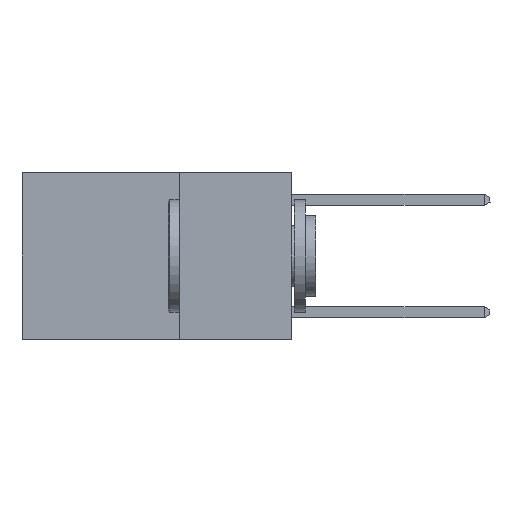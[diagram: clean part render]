
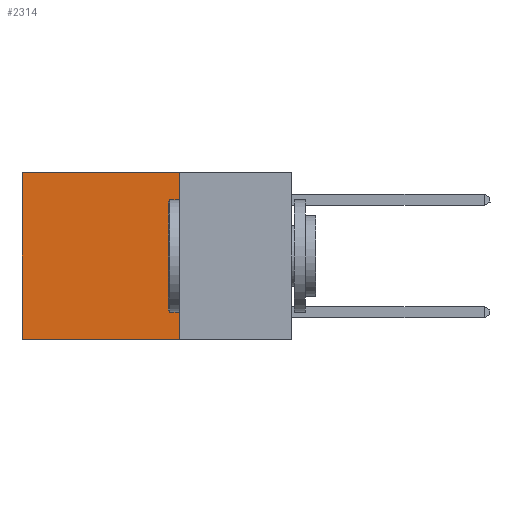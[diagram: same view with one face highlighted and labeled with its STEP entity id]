
A CAD part, left-side view. The second image highlights one B-rep face of the part: STEP entity #2314.
In plain terms, the highlighted planar face has unit normal (-1, 0, 0).
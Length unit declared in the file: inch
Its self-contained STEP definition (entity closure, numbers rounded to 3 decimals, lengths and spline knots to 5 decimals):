
#237 = PLANE ( 'NONE',  #12781 ) ;
#342 = CARTESIAN_POINT ( 'NONE',  ( 0.2625, 0.25, -0.37 ) ) ;
#918 = EDGE_CURVE ( 'NONE', #11127, #9048, #18905, .T. ) ;
#1229 = ORIENTED_EDGE ( 'NONE', *, *, #2737, .F. ) ;
#1987 = LINE ( 'NONE', #20059, #13210 ) ;
#2314 = ADVANCED_FACE ( 'NONE', ( #23925 ), #237, .F. ) ;
#2494 = ORIENTED_EDGE ( 'NONE', *, *, #918, .T. ) ;
#2737 = EDGE_CURVE ( 'NONE', #11127, #18868, #18816, .T. ) ;
#3712 = CARTESIAN_POINT ( 'NONE',  ( 0.2625, 0.25, -0.37 ) ) ;
#6930 = CARTESIAN_POINT ( 'NONE',  ( 0.2625, 0.25, 0. ) ) ;
#7854 = EDGE_CURVE ( 'NONE', #18868, #22643, #19022, .T. ) ;
#8993 = VECTOR ( 'NONE', #26523, 39.37008 ) ;
#9048 = VERTEX_POINT ( 'NONE', #21240 ) ;
#10449 = VECTOR ( 'NONE', #20209, 39.37008 ) ;
#10558 = VECTOR ( 'NONE', #26427, 39.37008 ) ;
#10932 = CARTESIAN_POINT ( 'NONE',  ( 0.2625, 0.6, -0.37 ) ) ;
#11127 = VERTEX_POINT ( 'NONE', #15451 ) ;
#11184 = DIRECTION ( 'NONE',  ( 1., 0., 0. ) ) ;
#11367 = CARTESIAN_POINT ( 'NONE',  ( 0.2625, 0.25, 0. ) ) ;
#11374 = DIRECTION ( 'NONE',  ( 0., 0., -1. ) ) ;
#12781 = AXIS2_PLACEMENT_3D ( 'NONE', #6930, #11184, #11374 ) ;
#13210 = VECTOR ( 'NONE', #26613, 39.37008 ) ;
#14506 = ORIENTED_EDGE ( 'NONE', *, *, #15100, .T. ) ;
#15100 = EDGE_CURVE ( 'NONE', #9048, #22643, #1987, .T. ) ;
#15451 = CARTESIAN_POINT ( 'NONE',  ( 0.2625, 0.25, 0. ) ) ;
#16544 = ORIENTED_EDGE ( 'NONE', *, *, #7854, .F. ) ;
#18022 = CARTESIAN_POINT ( 'NONE',  ( 0.2625, 0.25, 0. ) ) ;
#18816 = LINE ( 'NONE', #11367, #8993 ) ;
#18868 = VERTEX_POINT ( 'NONE', #3712 ) ;
#18905 = LINE ( 'NONE', #18022, #10449 ) ;
#19022 = LINE ( 'NONE', #342, #10558 ) ;
#20059 = CARTESIAN_POINT ( 'NONE',  ( 0.2625, 0.6, 0. ) ) ;
#20209 = DIRECTION ( 'NONE',  ( 0., 1., 0. ) ) ;
#21240 = CARTESIAN_POINT ( 'NONE',  ( 0.2625, 0.6, 0. ) ) ;
#22643 = VERTEX_POINT ( 'NONE', #10932 ) ;
#23925 = FACE_OUTER_BOUND ( 'NONE', #24531, .T. ) ;
#24531 = EDGE_LOOP ( 'NONE', ( #14506, #16544, #1229, #2494 ) ) ;
#26427 = DIRECTION ( 'NONE',  ( 0., 1., 0. ) ) ;
#26523 = DIRECTION ( 'NONE',  ( 0., 0., -1. ) ) ;
#26613 = DIRECTION ( 'NONE',  ( 0., 0., -1. ) ) ;
